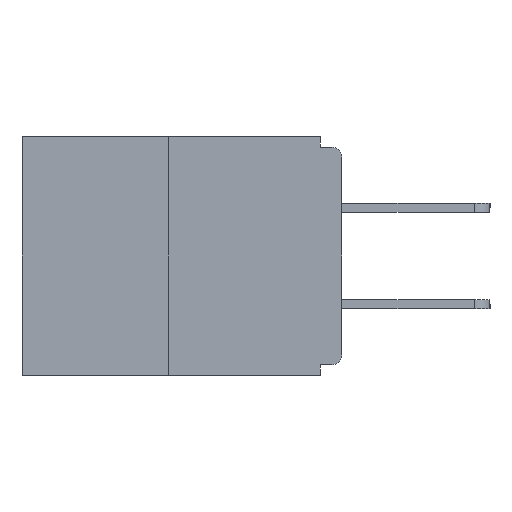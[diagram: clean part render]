
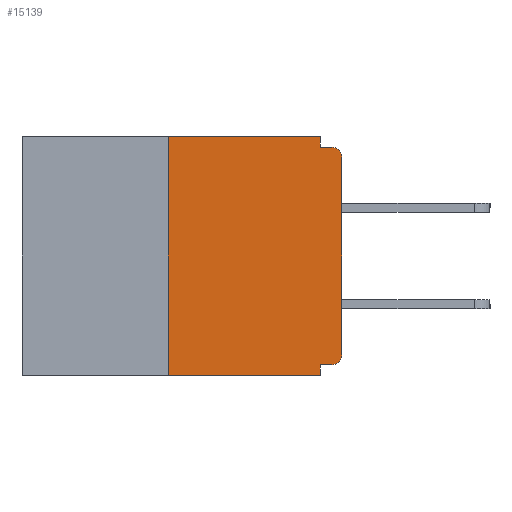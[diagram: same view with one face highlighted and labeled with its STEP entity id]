
A CAD part, left-side view. The second image highlights one B-rep face of the part: STEP entity #15139.
In plain terms, the highlighted planar face has unit normal (-1, 0, 0).
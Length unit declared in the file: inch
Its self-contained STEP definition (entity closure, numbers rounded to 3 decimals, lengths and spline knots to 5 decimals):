
#173 = CARTESIAN_POINT ( 'NONE',  ( 0., 0.015, -0.03 ) ) ;
#204 = EDGE_CURVE ( 'NONE', #14257, #12609, #2890, .T. ) ;
#472 = VERTEX_POINT ( 'NONE', #10508 ) ;
#699 = DIRECTION ( 'NONE',  ( 0., 0., -1. ) ) ;
#757 = ORIENTED_EDGE ( 'NONE', *, *, #6935, .T. ) ;
#827 = CARTESIAN_POINT ( 'NONE',  ( 0., 0., -0.03 ) ) ;
#1043 = LINE ( 'NONE', #5183, #7671 ) ;
#1210 = PLANE ( 'NONE',  #7931 ) ;
#1274 = ORIENTED_EDGE ( 'NONE', *, *, #10219, .F. ) ;
#1330 = CARTESIAN_POINT ( 'NONE',  ( 0., 0.46, 0. ) ) ;
#1902 = CARTESIAN_POINT ( 'NONE',  ( 0., 0.031, 0. ) ) ;
#1933 = CARTESIAN_POINT ( 'NONE',  ( 0., 0.031, -0.015 ) ) ;
#1960 = EDGE_LOOP ( 'NONE', ( #10993, #7766, #8590, #14377, #1274, #2243, #757, #2887, #13712, #2773 ) ) ;
#2155 = VERTEX_POINT ( 'NONE', #3745 ) ;
#2243 = ORIENTED_EDGE ( 'NONE', *, *, #204, .T. ) ;
#2328 = EDGE_CURVE ( 'NONE', #3622, #2155, #5470, .T. ) ;
#2384 = VECTOR ( 'NONE', #13470, 39.37008 ) ;
#2456 = CIRCLE ( 'NONE', #4352, 0.015 ) ;
#2773 = ORIENTED_EDGE ( 'NONE', *, *, #6789, .F. ) ;
#2887 = ORIENTED_EDGE ( 'NONE', *, *, #14794, .T. ) ;
#2890 = CIRCLE ( 'NONE', #8964, 0.015 ) ;
#3145 = DIRECTION ( 'NONE',  ( -1., 0., 0. ) ) ;
#3155 = CARTESIAN_POINT ( 'NONE',  ( 0., 0.031, -0.343 ) ) ;
#3222 = LINE ( 'NONE', #5260, #8010 ) ;
#3333 = DIRECTION ( 'NONE',  ( 0., 1., 0. ) ) ;
#3622 = VERTEX_POINT ( 'NONE', #15611 ) ;
#3745 = CARTESIAN_POINT ( 'NONE',  ( 0., 0.031, -0.343 ) ) ;
#3974 = DIRECTION ( 'NONE',  ( 0., 0., 1. ) ) ;
#4094 = DIRECTION ( 'NONE',  ( 1., 0., 0. ) ) ;
#4352 = AXIS2_PLACEMENT_3D ( 'NONE', #173, #8119, #6805 ) ;
#5131 = VERTEX_POINT ( 'NONE', #1902 ) ;
#5183 = CARTESIAN_POINT ( 'NONE',  ( 0., 0.46, 0. ) ) ;
#5260 = CARTESIAN_POINT ( 'NONE',  ( 0., 0., 0. ) ) ;
#5364 = VECTOR ( 'NONE', #16875, 39.37008 ) ;
#5470 = LINE ( 'NONE', #3155, #16553 ) ;
#5593 = EDGE_CURVE ( 'NONE', #472, #5131, #1043, .T. ) ;
#6272 = CARTESIAN_POINT ( 'NONE',  ( 0., 0., -0.313 ) ) ;
#6445 = CARTESIAN_POINT ( 'NONE',  ( 0., 0., -0.015 ) ) ;
#6511 = EDGE_CURVE ( 'NONE', #11849, #472, #10667, .T. ) ;
#6789 = EDGE_CURVE ( 'NONE', #5131, #10558, #13315, .T. ) ;
#6805 = DIRECTION ( 'NONE',  ( 0., 0., -1. ) ) ;
#6935 = EDGE_CURVE ( 'NONE', #12609, #13830, #3222, .T. ) ;
#7081 = LINE ( 'NONE', #9749, #13576 ) ;
#7671 = VECTOR ( 'NONE', #13157, 39.37008 ) ;
#7766 = ORIENTED_EDGE ( 'NONE', *, *, #6511, .F. ) ;
#7931 = AXIS2_PLACEMENT_3D ( 'NONE', #1330, #4094, #10440 ) ;
#7943 = EDGE_CURVE ( 'NONE', #11849, #2155, #16126, .T. ) ;
#8010 = VECTOR ( 'NONE', #3974, 39.37008 ) ;
#8013 = CARTESIAN_POINT ( 'NONE',  ( 0., 0.015, -0.328 ) ) ;
#8119 = DIRECTION ( 'NONE',  ( -1., 0., 0. ) ) ;
#8343 = CARTESIAN_POINT ( 'NONE',  ( 0., 0.46, -0.343 ) ) ;
#8590 = ORIENTED_EDGE ( 'NONE', *, *, #7943, .T. ) ;
#8964 = AXIS2_PLACEMENT_3D ( 'NONE', #12342, #3145, #9738 ) ;
#9134 = CARTESIAN_POINT ( 'NONE',  ( 0., 0.015, -0.015 ) ) ;
#9738 = DIRECTION ( 'NONE',  ( 0., 0., -1. ) ) ;
#9749 = CARTESIAN_POINT ( 'NONE',  ( 0., 0., -0.328 ) ) ;
#9852 = VECTOR ( 'NONE', #14134, 39.37008 ) ;
#10219 = EDGE_CURVE ( 'NONE', #14257, #3622, #7081, .T. ) ;
#10440 = DIRECTION ( 'NONE',  ( 0., 0., -1. ) ) ;
#10508 = CARTESIAN_POINT ( 'NONE',  ( 0., 0.25, 0. ) ) ;
#10558 = VERTEX_POINT ( 'NONE', #1933 ) ;
#10667 = LINE ( 'NONE', #14353, #10855 ) ;
#10855 = VECTOR ( 'NONE', #15600, 39.37008 ) ;
#10993 = ORIENTED_EDGE ( 'NONE', *, *, #5593, .F. ) ;
#11116 = LINE ( 'NONE', #6445, #5364 ) ;
#11138 = EDGE_CURVE ( 'NONE', #10558, #12822, #11116, .T. ) ;
#11849 = VERTEX_POINT ( 'NONE', #16469 ) ;
#12342 = CARTESIAN_POINT ( 'NONE',  ( 0., 0.015, -0.313 ) ) ;
#12609 = VERTEX_POINT ( 'NONE', #6272 ) ;
#12822 = VERTEX_POINT ( 'NONE', #9134 ) ;
#13056 = CARTESIAN_POINT ( 'NONE',  ( 0., 0.031, 0. ) ) ;
#13157 = DIRECTION ( 'NONE',  ( 0., -1., 0. ) ) ;
#13315 = LINE ( 'NONE', #13056, #9852 ) ;
#13321 = FACE_OUTER_BOUND ( 'NONE', #1960, .T. ) ;
#13470 = DIRECTION ( 'NONE',  ( 0., -1., 0. ) ) ;
#13576 = VECTOR ( 'NONE', #3333, 39.37008 ) ;
#13712 = ORIENTED_EDGE ( 'NONE', *, *, #11138, .F. ) ;
#13830 = VERTEX_POINT ( 'NONE', #827 ) ;
#14134 = DIRECTION ( 'NONE',  ( 0., 0., -1. ) ) ;
#14257 = VERTEX_POINT ( 'NONE', #8013 ) ;
#14353 = CARTESIAN_POINT ( 'NONE',  ( 0., 0.25, 0. ) ) ;
#14377 = ORIENTED_EDGE ( 'NONE', *, *, #2328, .F. ) ;
#14794 = EDGE_CURVE ( 'NONE', #13830, #12822, #2456, .T. ) ;
#15139 = ADVANCED_FACE ( 'NONE', ( #13321 ), #1210, .F. ) ;
#15600 = DIRECTION ( 'NONE',  ( 0., 0., 1. ) ) ;
#15611 = CARTESIAN_POINT ( 'NONE',  ( 0., 0.031, -0.328 ) ) ;
#16126 = LINE ( 'NONE', #8343, #2384 ) ;
#16469 = CARTESIAN_POINT ( 'NONE',  ( 0., 0.25, -0.343 ) ) ;
#16553 = VECTOR ( 'NONE', #699, 39.37008 ) ;
#16875 = DIRECTION ( 'NONE',  ( 0., -1., 0. ) ) ;
